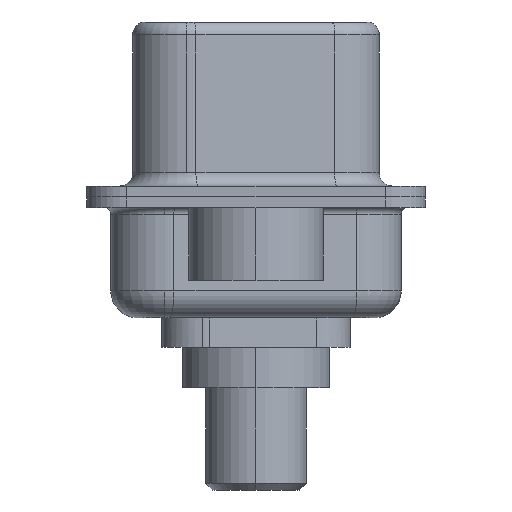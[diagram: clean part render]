
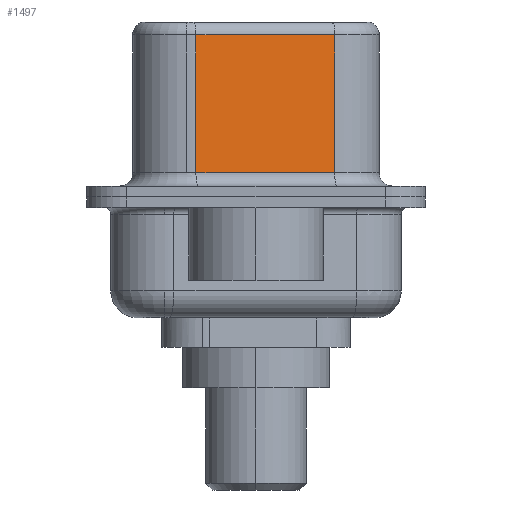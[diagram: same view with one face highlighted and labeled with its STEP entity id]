
A CAD part, left-side view. The second image highlights one B-rep face of the part: STEP entity #1497.
In plain terms, the highlighted planar face has unit normal (-0.985, -0.174, 0).
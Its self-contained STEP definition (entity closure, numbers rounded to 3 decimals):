
#179 = ORIENTED_EDGE ( 'NONE', *, *, #16501, .T. ) ;
#409 = CARTESIAN_POINT ( 'NONE',  ( 3.675, 2.233, 6.52 ) ) ;
#1497 = ADVANCED_FACE ( 'NONE', ( #13563 ), #13989, .F. ) ;
#1575 = CARTESIAN_POINT ( 'NONE',  ( 4.585, -2.927, 6.02 ) ) ;
#2553 = CARTESIAN_POINT ( 'NONE',  ( 4.585, -2.927, 0.9 ) ) ;
#2920 = DIRECTION ( 'NONE',  ( -0.174, 0.985, 0. ) ) ;
#3219 = ORIENTED_EDGE ( 'NONE', *, *, #12467, .T. ) ;
#3636 = CARTESIAN_POINT ( 'NONE',  ( 4.585, -2.927, 6.52 ) ) ;
#5134 = EDGE_CURVE ( 'NONE', #5359, #12226, #9454, .T. ) ;
#5214 = DIRECTION ( 'NONE',  ( 0.174, -0.985, 0. ) ) ;
#5359 = VERTEX_POINT ( 'NONE', #8207 ) ;
#7105 = CARTESIAN_POINT ( 'NONE',  ( 3.675, 2.233, 6.02 ) ) ;
#8072 = VECTOR ( 'NONE', #14905, 1000. ) ;
#8101 = VERTEX_POINT ( 'NONE', #12404 ) ;
#8207 = CARTESIAN_POINT ( 'NONE',  ( 4.585, -2.927, 6.02 ) ) ;
#8851 = LINE ( 'NONE', #1575, #15433 ) ;
#9166 = DIRECTION ( 'NONE',  ( 0., 0., -1. ) ) ;
#9342 = VECTOR ( 'NONE', #5214, 1000. ) ;
#9454 = LINE ( 'NONE', #16875, #16872 ) ;
#11648 = ORIENTED_EDGE ( 'NONE', *, *, #5134, .F. ) ;
#12226 = VERTEX_POINT ( 'NONE', #12708 ) ;
#12404 = CARTESIAN_POINT ( 'NONE',  ( 3.675, 2.233, 0.9 ) ) ;
#12467 = EDGE_CURVE ( 'NONE', #8101, #12226, #12836, .T. ) ;
#12708 = CARTESIAN_POINT ( 'NONE',  ( 4.585, -2.927, 0.9 ) ) ;
#12836 = LINE ( 'NONE', #2553, #9342 ) ;
#13185 = DIRECTION ( 'NONE',  ( -0.174, 0.985, 0. ) ) ;
#13563 = FACE_OUTER_BOUND ( 'NONE', #13729, .T. ) ;
#13617 = EDGE_CURVE ( 'NONE', #13731, #8101, #15698, .T. ) ;
#13729 = EDGE_LOOP ( 'NONE', ( #11648, #179, #15217, #3219 ) ) ;
#13731 = VERTEX_POINT ( 'NONE', #7105 ) ;
#13932 = DIRECTION ( 'NONE',  ( 0.985, 0.174, 0. ) ) ;
#13989 = PLANE ( 'NONE',  #14483 ) ;
#14483 = AXIS2_PLACEMENT_3D ( 'NONE', #3636, #13932, #13185 ) ;
#14905 = DIRECTION ( 'NONE',  ( 0., 0., -1. ) ) ;
#15217 = ORIENTED_EDGE ( 'NONE', *, *, #13617, .T. ) ;
#15433 = VECTOR ( 'NONE', #2920, 1000. ) ;
#15698 = LINE ( 'NONE', #409, #8072 ) ;
#16501 = EDGE_CURVE ( 'NONE', #5359, #13731, #8851, .T. ) ;
#16872 = VECTOR ( 'NONE', #9166, 1000. ) ;
#16875 = CARTESIAN_POINT ( 'NONE',  ( 4.585, -2.927, 6.52 ) ) ;
